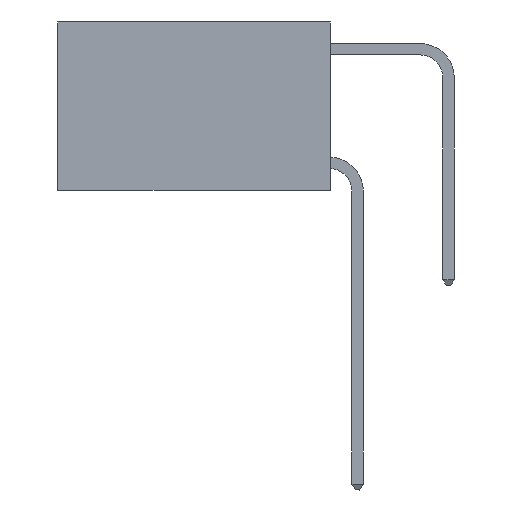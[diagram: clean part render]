
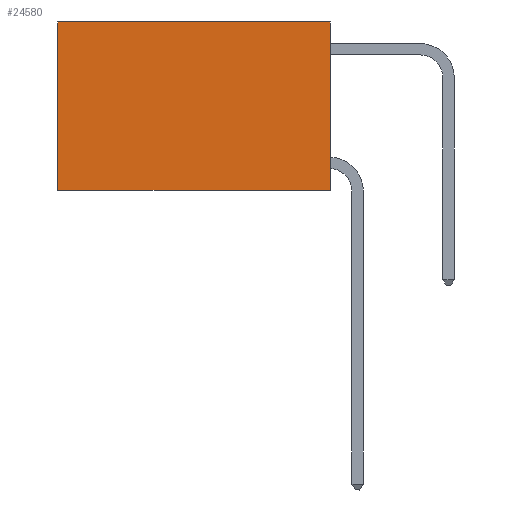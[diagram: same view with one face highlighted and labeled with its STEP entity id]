
A CAD part, left-side view. The second image highlights one B-rep face of the part: STEP entity #24580.
In plain terms, the highlighted planar face has unit normal (-1, 0, 0).
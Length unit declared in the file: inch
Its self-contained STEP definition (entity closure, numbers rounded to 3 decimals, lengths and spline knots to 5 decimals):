
#152 = DIRECTION ( 'NONE',  ( 0., 0., -1. ) ) ;
#694 = EDGE_CURVE ( 'NONE', #21440, #2020, #11006, .T. ) ;
#2020 = VERTEX_POINT ( 'NONE', #21531 ) ;
#2043 = VECTOR ( 'NONE', #152, 39.37008 ) ;
#3499 = AXIS2_PLACEMENT_3D ( 'NONE', #5286, #9293, #5630 ) ;
#4789 = CARTESIAN_POINT ( 'NONE',  ( 0.2625, 0., 0. ) ) ;
#5286 = CARTESIAN_POINT ( 'NONE',  ( 0.2625, 0., 0. ) ) ;
#5358 = CARTESIAN_POINT ( 'NONE',  ( 0.2625, 0.6, -0.37 ) ) ;
#5630 = DIRECTION ( 'NONE',  ( 0., 0., -1. ) ) ;
#7114 = CARTESIAN_POINT ( 'NONE',  ( 0.2625, 0.6, 0. ) ) ;
#7314 = EDGE_CURVE ( 'NONE', #10809, #20313, #12750, .T. ) ;
#7607 = CARTESIAN_POINT ( 'NONE',  ( 0.2625, 0.6, 0. ) ) ;
#7877 = ORIENTED_EDGE ( 'NONE', *, *, #24778, .F. ) ;
#7954 = DIRECTION ( 'NONE',  ( 0., 1., 0. ) ) ;
#8871 = VECTOR ( 'NONE', #17477, 39.37008 ) ;
#9293 = DIRECTION ( 'NONE',  ( 1., 0., 0. ) ) ;
#10809 = VERTEX_POINT ( 'NONE', #7114 ) ;
#11006 = LINE ( 'NONE', #4789, #15817 ) ;
#11792 = LINE ( 'NONE', #19408, #21095 ) ;
#12616 = ORIENTED_EDGE ( 'NONE', *, *, #694, .F. ) ;
#12750 = LINE ( 'NONE', #7607, #2043 ) ;
#13895 = EDGE_LOOP ( 'NONE', ( #23328, #7877, #12616, #23373 ) ) ;
#15817 = VECTOR ( 'NONE', #18158, 39.37008 ) ;
#17477 = DIRECTION ( 'NONE',  ( 0., 1., 0. ) ) ;
#17643 = CARTESIAN_POINT ( 'NONE',  ( 0.2625, 0., 0. ) ) ;
#18158 = DIRECTION ( 'NONE',  ( 0., 0., -1. ) ) ;
#19408 = CARTESIAN_POINT ( 'NONE',  ( 0.2625, 0., -0.37 ) ) ;
#19954 = EDGE_CURVE ( 'NONE', #21440, #10809, #23561, .T. ) ;
#20196 = FACE_OUTER_BOUND ( 'NONE', #13895, .T. ) ;
#20313 = VERTEX_POINT ( 'NONE', #5358 ) ;
#21095 = VECTOR ( 'NONE', #7954, 39.37008 ) ;
#21440 = VERTEX_POINT ( 'NONE', #22639 ) ;
#21531 = CARTESIAN_POINT ( 'NONE',  ( 0.2625, 0., -0.37 ) ) ;
#22639 = CARTESIAN_POINT ( 'NONE',  ( 0.2625, 0., 0. ) ) ;
#22748 = PLANE ( 'NONE',  #3499 ) ;
#23328 = ORIENTED_EDGE ( 'NONE', *, *, #7314, .T. ) ;
#23373 = ORIENTED_EDGE ( 'NONE', *, *, #19954, .T. ) ;
#23561 = LINE ( 'NONE', #17643, #8871 ) ;
#24580 = ADVANCED_FACE ( 'NONE', ( #20196 ), #22748, .F. ) ;
#24778 = EDGE_CURVE ( 'NONE', #2020, #20313, #11792, .T. ) ;
